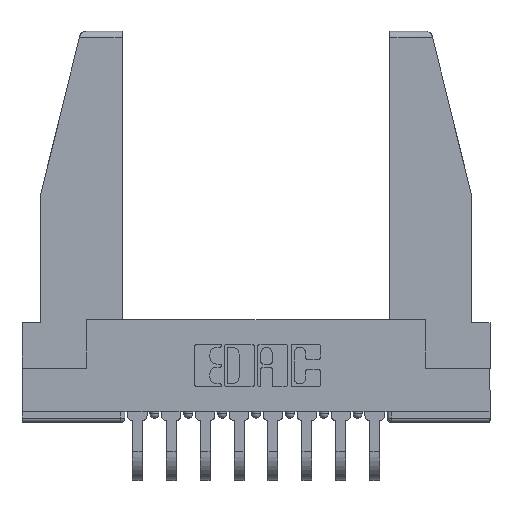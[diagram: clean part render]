
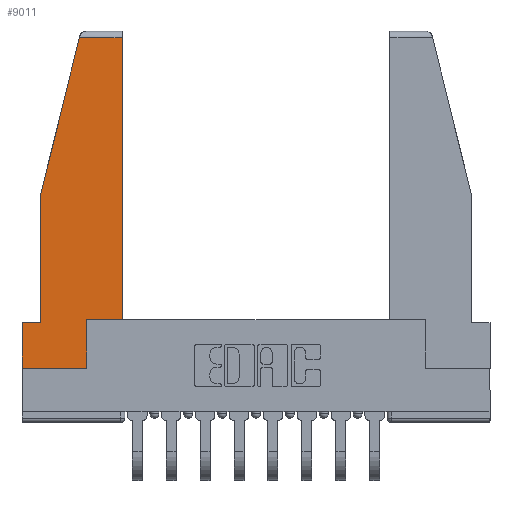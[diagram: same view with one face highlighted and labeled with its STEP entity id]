
A CAD part, top view. The second image highlights one B-rep face of the part: STEP entity #9011.
In plain terms, the highlighted planar face has unit normal (0, 0, 1).
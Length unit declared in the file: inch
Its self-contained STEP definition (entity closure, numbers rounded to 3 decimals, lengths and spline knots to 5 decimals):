
#49 = VECTOR ( 'NONE', #827, 39.37008 ) ;
#238 = CARTESIAN_POINT ( 'NONE',  ( 0.2636, 1.52, 0. ) ) ;
#322 = VECTOR ( 'NONE', #5260, 39.37008 ) ;
#540 = FACE_OUTER_BOUND ( 'NONE', #623, .T. ) ;
#623 = EDGE_LOOP ( 'NONE', ( #13392, #6510, #1799, #11432, #10443, #3138, #5524, #7279, #6104 ) ) ;
#752 = CARTESIAN_POINT ( 'NONE',  ( 0.271, 1.55, 0. ) ) ;
#827 = DIRECTION ( 'NONE',  ( -0.239, -0.971, 0. ) ) ;
#845 = LINE ( 'NONE', #3049, #6262 ) ;
#857 = EDGE_CURVE ( 'NONE', #7233, #10685, #4152, .T. ) ;
#906 = DIRECTION ( 'NONE',  ( -1., 0., 0. ) ) ;
#1043 = VECTOR ( 'NONE', #3974, 39.37008 ) ;
#1577 = CARTESIAN_POINT ( 'NONE',  ( 0., 0., 0. ) ) ;
#1799 = ORIENTED_EDGE ( 'NONE', *, *, #6112, .T. ) ;
#2084 = VECTOR ( 'NONE', #3791, 39.37008 ) ;
#2160 = VERTEX_POINT ( 'NONE', #12702 ) ;
#2222 = VERTEX_POINT ( 'NONE', #9778 ) ;
#2738 = CARTESIAN_POINT ( 'NONE',  ( 0.461, 1.52, 0. ) ) ;
#2848 = EDGE_CURVE ( 'NONE', #10685, #5319, #845, .T. ) ;
#2885 = EDGE_CURVE ( 'NONE', #2222, #6737, #3957, .T. ) ;
#3049 = CARTESIAN_POINT ( 'NONE',  ( 0.461, 0.223, 0. ) ) ;
#3138 = ORIENTED_EDGE ( 'NONE', *, *, #10389, .T. ) ;
#3513 = DIRECTION ( 'NONE',  ( 0., 0., 1. ) ) ;
#3791 = DIRECTION ( 'NONE',  ( 0., -1., 0. ) ) ;
#3907 = VECTOR ( 'NONE', #4353, 39.37008 ) ;
#3957 = LINE ( 'NONE', #7104, #11583 ) ;
#3974 = DIRECTION ( 'NONE',  ( -1., 0., 0. ) ) ;
#4124 = CARTESIAN_POINT ( 'NONE',  ( 0.086, 0.8, 0. ) ) ;
#4152 = LINE ( 'NONE', #12590, #3907 ) ;
#4353 = DIRECTION ( 'NONE',  ( 1., 0., 0. ) ) ;
#4623 = LINE ( 'NONE', #6291, #322 ) ;
#4684 = DIRECTION ( 'NONE',  ( 0., -1., 0. ) ) ;
#4763 = CARTESIAN_POINT ( 'NONE',  ( 0., 0., 0. ) ) ;
#5048 = VERTEX_POINT ( 'NONE', #4124 ) ;
#5260 = DIRECTION ( 'NONE',  ( 1., 0., 0. ) ) ;
#5275 = EDGE_CURVE ( 'NONE', #5319, #12524, #13229, .T. ) ;
#5319 = VERTEX_POINT ( 'NONE', #2738 ) ;
#5524 = ORIENTED_EDGE ( 'NONE', *, *, #12890, .T. ) ;
#5857 = LINE ( 'NONE', #8130, #2084 ) ;
#6004 = DIRECTION ( 'NONE',  ( 0., 1., 0. ) ) ;
#6104 = ORIENTED_EDGE ( 'NONE', *, *, #857, .T. ) ;
#6112 = EDGE_CURVE ( 'NONE', #12524, #5048, #10281, .T. ) ;
#6262 = VECTOR ( 'NONE', #6004, 39.37008 ) ;
#6291 = CARTESIAN_POINT ( 'NONE',  ( 0., 0., 0. ) ) ;
#6510 = ORIENTED_EDGE ( 'NONE', *, *, #5275, .T. ) ;
#6513 = VECTOR ( 'NONE', #4684, 39.37008 ) ;
#6523 = CARTESIAN_POINT ( 'NONE',  ( 0.461, 0.223, 0. ) ) ;
#6737 = VERTEX_POINT ( 'NONE', #9893 ) ;
#7104 = CARTESIAN_POINT ( 'NONE',  ( 0., 0.21, 0. ) ) ;
#7132 = DIRECTION ( 'NONE',  ( 0., 1., 0. ) ) ;
#7233 = VERTEX_POINT ( 'NONE', #13046 ) ;
#7279 = ORIENTED_EDGE ( 'NONE', *, *, #13566, .T. ) ;
#7390 = VECTOR ( 'NONE', #7132, 39.37008 ) ;
#8130 = CARTESIAN_POINT ( 'NONE',  ( 0.086, 0.8, 0. ) ) ;
#8434 = CARTESIAN_POINT ( 'NONE',  ( 0.297, 0., 0. ) ) ;
#8911 = AXIS2_PLACEMENT_3D ( 'NONE', #4763, #3513, #8957 ) ;
#8957 = DIRECTION ( 'NONE',  ( 1., 0., 0. ) ) ;
#9011 = ADVANCED_FACE ( 'NONE', ( #540 ), #10827, .T. ) ;
#9778 = CARTESIAN_POINT ( 'NONE',  ( 0.086, 0.21, 0. ) ) ;
#9893 = CARTESIAN_POINT ( 'NONE',  ( 0., 0.21, 0. ) ) ;
#10056 = CARTESIAN_POINT ( 'NONE',  ( 0., 1.52, 0. ) ) ;
#10135 = LINE ( 'NONE', #12299, #6513 ) ;
#10281 = LINE ( 'NONE', #752, #49 ) ;
#10389 = EDGE_CURVE ( 'NONE', #6737, #12195, #10135, .T. ) ;
#10443 = ORIENTED_EDGE ( 'NONE', *, *, #2885, .T. ) ;
#10534 = LINE ( 'NONE', #8434, #7390 ) ;
#10685 = VERTEX_POINT ( 'NONE', #6523 ) ;
#10827 = PLANE ( 'NONE',  #8911 ) ;
#11432 = ORIENTED_EDGE ( 'NONE', *, *, #12957, .T. ) ;
#11583 = VECTOR ( 'NONE', #906, 39.37008 ) ;
#12195 = VERTEX_POINT ( 'NONE', #1577 ) ;
#12299 = CARTESIAN_POINT ( 'NONE',  ( 0., 0.21, 0. ) ) ;
#12524 = VERTEX_POINT ( 'NONE', #238 ) ;
#12590 = CARTESIAN_POINT ( 'NONE',  ( 0.297, 0.223, 0. ) ) ;
#12702 = CARTESIAN_POINT ( 'NONE',  ( 0.297, 0., 0. ) ) ;
#12890 = EDGE_CURVE ( 'NONE', #12195, #2160, #4623, .T. ) ;
#12957 = EDGE_CURVE ( 'NONE', #5048, #2222, #5857, .T. ) ;
#13046 = CARTESIAN_POINT ( 'NONE',  ( 0.297, 0.223, 0. ) ) ;
#13229 = LINE ( 'NONE', #10056, #1043 ) ;
#13392 = ORIENTED_EDGE ( 'NONE', *, *, #2848, .T. ) ;
#13566 = EDGE_CURVE ( 'NONE', #2160, #7233, #10534, .T. ) ;
